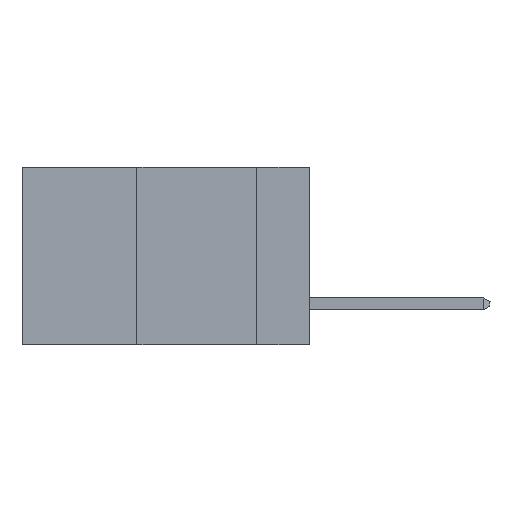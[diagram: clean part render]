
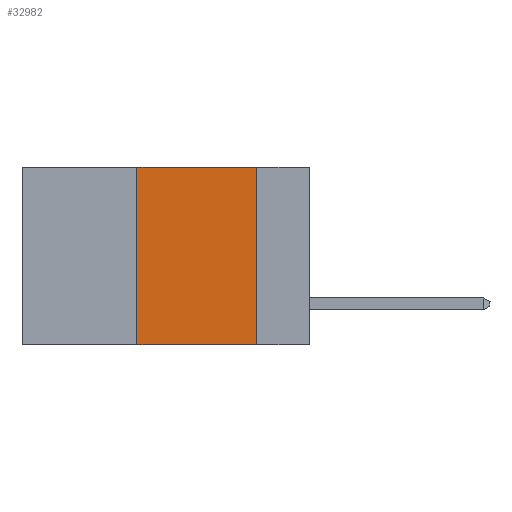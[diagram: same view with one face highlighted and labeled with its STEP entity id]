
A CAD part, left-side view. The second image highlights one B-rep face of the part: STEP entity #32982.
In plain terms, the highlighted planar face has unit normal (-1, 0, 0).
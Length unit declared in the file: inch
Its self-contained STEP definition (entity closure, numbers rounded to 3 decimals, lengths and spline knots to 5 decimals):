
#2751 = LINE ( 'NONE', #19870, #19798 ) ;
#2977 = DIRECTION ( 'NONE',  ( 0., 0., -1. ) ) ;
#4655 = AXIS2_PLACEMENT_3D ( 'NONE', #16822, #13699, #30356 ) ;
#6368 = FACE_OUTER_BOUND ( 'NONE', #40317, .T. ) ;
#7017 = PLANE ( 'NONE',  #4655 ) ;
#9506 = CARTESIAN_POINT ( 'NONE',  ( 0., 0.36, -0.37 ) ) ;
#12405 = EDGE_CURVE ( 'NONE', #26288, #32279, #38368, .T. ) ;
#13699 = DIRECTION ( 'NONE',  ( 1., 0., 0. ) ) ;
#14946 = CARTESIAN_POINT ( 'NONE',  ( 0., 0.11, -0.37 ) ) ;
#15558 = CARTESIAN_POINT ( 'NONE',  ( 0., 0.36, 0. ) ) ;
#16166 = ORIENTED_EDGE ( 'NONE', *, *, #37565, .F. ) ;
#16822 = CARTESIAN_POINT ( 'NONE',  ( 0., 0.6, 0. ) ) ;
#17639 = CARTESIAN_POINT ( 'NONE',  ( 0., 0.11, 0. ) ) ;
#18386 = LINE ( 'NONE', #31935, #20987 ) ;
#19798 = VECTOR ( 'NONE', #2977, 39.37008 ) ;
#19870 = CARTESIAN_POINT ( 'NONE',  ( 0., 0.11, 0. ) ) ;
#20357 = CARTESIAN_POINT ( 'NONE',  ( 0., 0.6, -0.37 ) ) ;
#20571 = LINE ( 'NONE', #20357, #32047 ) ;
#20987 = VECTOR ( 'NONE', #42164, 39.37008 ) ;
#21407 = EDGE_CURVE ( 'NONE', #26288, #38401, #20571, .T. ) ;
#24600 = CARTESIAN_POINT ( 'NONE',  ( 0., 0.36, 0. ) ) ;
#26288 = VERTEX_POINT ( 'NONE', #9506 ) ;
#30133 = DIRECTION ( 'NONE',  ( 0., -1., 0. ) ) ;
#30356 = DIRECTION ( 'NONE',  ( 0., 0., -1. ) ) ;
#30598 = DIRECTION ( 'NONE',  ( 0., 0., 1. ) ) ;
#31451 = EDGE_CURVE ( 'NONE', #32279, #33494, #18386, .T. ) ;
#31935 = CARTESIAN_POINT ( 'NONE',  ( 0., 0.6, 0. ) ) ;
#32047 = VECTOR ( 'NONE', #30133, 39.37008 ) ;
#32279 = VERTEX_POINT ( 'NONE', #15558 ) ;
#32982 = ADVANCED_FACE ( 'NONE', ( #6368 ), #7017, .F. ) ;
#33494 = VERTEX_POINT ( 'NONE', #17639 ) ;
#36016 = ORIENTED_EDGE ( 'NONE', *, *, #31451, .F. ) ;
#37565 = EDGE_CURVE ( 'NONE', #33494, #38401, #2751, .T. ) ;
#38368 = LINE ( 'NONE', #24600, #38916 ) ;
#38401 = VERTEX_POINT ( 'NONE', #14946 ) ;
#38916 = VECTOR ( 'NONE', #30598, 39.37008 ) ;
#40317 = EDGE_LOOP ( 'NONE', ( #16166, #36016, #42451, #40430 ) ) ;
#40430 = ORIENTED_EDGE ( 'NONE', *, *, #21407, .T. ) ;
#42164 = DIRECTION ( 'NONE',  ( 0., -1., 0. ) ) ;
#42451 = ORIENTED_EDGE ( 'NONE', *, *, #12405, .F. ) ;
